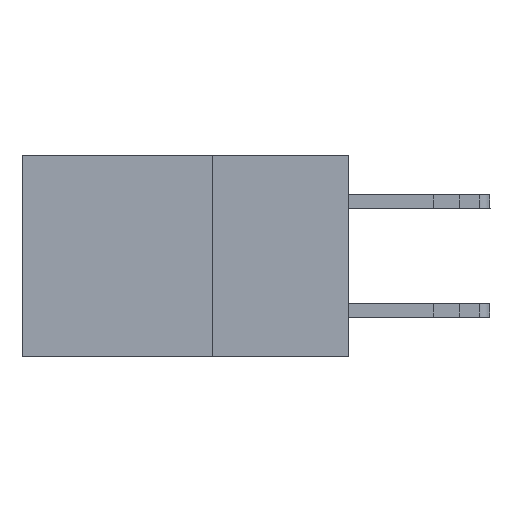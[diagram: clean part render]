
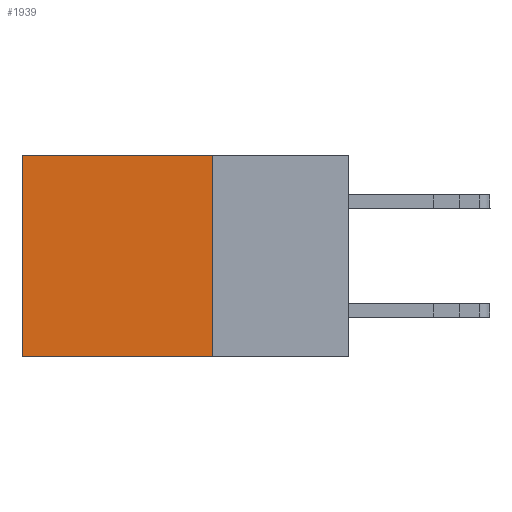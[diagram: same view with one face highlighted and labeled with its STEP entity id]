
A CAD part, left-side view. The second image highlights one B-rep face of the part: STEP entity #1939.
In plain terms, the highlighted planar face has unit normal (-1, 0, 0).
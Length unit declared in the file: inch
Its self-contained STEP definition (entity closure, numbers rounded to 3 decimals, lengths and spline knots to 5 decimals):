
#915 = CARTESIAN_POINT ( 'NONE',  ( 0.2615, 0.6, 0. ) ) ;
#1012 = VERTEX_POINT ( 'NONE', #915 ) ;
#1351 = DIRECTION ( 'NONE',  ( 0., 0., -1. ) ) ;
#1939 = ADVANCED_FACE ( 'NONE', ( #19668 ), #16979, .F. ) ;
#2074 = VECTOR ( 'NONE', #16151, 39.37008 ) ;
#2883 = CARTESIAN_POINT ( 'NONE',  ( 0.2615, 0.25, -0.37 ) ) ;
#3859 = ORIENTED_EDGE ( 'NONE', *, *, #13751, .T. ) ;
#4636 = ORIENTED_EDGE ( 'NONE', *, *, #5853, .F. ) ;
#4905 = AXIS2_PLACEMENT_3D ( 'NONE', #2883, #9135, #1351 ) ;
#5193 = CARTESIAN_POINT ( 'NONE',  ( 0.2615, 0.25, -0.37 ) ) ;
#5853 = EDGE_CURVE ( 'NONE', #20071, #15268, #13018, .T. ) ;
#5973 = CARTESIAN_POINT ( 'NONE',  ( 0.2615, 0.25, -0.37 ) ) ;
#6361 = CARTESIAN_POINT ( 'NONE',  ( 0.2615, 0.25, 0. ) ) ;
#9135 = DIRECTION ( 'NONE',  ( 1., 0., 0. ) ) ;
#9175 = EDGE_CURVE ( 'NONE', #15268, #10277, #20096, .T. ) ;
#10263 = CARTESIAN_POINT ( 'NONE',  ( 0.2615, 0.25, 0. ) ) ;
#10277 = VERTEX_POINT ( 'NONE', #17541 ) ;
#10577 = VECTOR ( 'NONE', #20102, 39.37008 ) ;
#10814 = CARTESIAN_POINT ( 'NONE',  ( 0.2615, 0.6, -0.37 ) ) ;
#11015 = ORIENTED_EDGE ( 'NONE', *, *, #16785, .T. ) ;
#11520 = LINE ( 'NONE', #6361, #2074 ) ;
#12437 = VECTOR ( 'NONE', #18556, 39.37008 ) ;
#13018 = LINE ( 'NONE', #5193, #17327 ) ;
#13751 = EDGE_CURVE ( 'NONE', #1012, #10277, #18565, .T. ) ;
#15268 = VERTEX_POINT ( 'NONE', #15750 ) ;
#15750 = CARTESIAN_POINT ( 'NONE',  ( 0.2615, 0.25, -0.37 ) ) ;
#16151 = DIRECTION ( 'NONE',  ( 0., 1., 0. ) ) ;
#16785 = EDGE_CURVE ( 'NONE', #20071, #1012, #11520, .T. ) ;
#16979 = PLANE ( 'NONE',  #4905 ) ;
#17327 = VECTOR ( 'NONE', #17760, 39.37008 ) ;
#17358 = EDGE_LOOP ( 'NONE', ( #3859, #17936, #4636, #11015 ) ) ;
#17541 = CARTESIAN_POINT ( 'NONE',  ( 0.2615, 0.6, -0.37 ) ) ;
#17760 = DIRECTION ( 'NONE',  ( 0., 0., -1. ) ) ;
#17936 = ORIENTED_EDGE ( 'NONE', *, *, #9175, .F. ) ;
#18556 = DIRECTION ( 'NONE',  ( 0., 1., 0. ) ) ;
#18565 = LINE ( 'NONE', #10814, #10577 ) ;
#19668 = FACE_OUTER_BOUND ( 'NONE', #17358, .T. ) ;
#20071 = VERTEX_POINT ( 'NONE', #10263 ) ;
#20096 = LINE ( 'NONE', #5973, #12437 ) ;
#20102 = DIRECTION ( 'NONE',  ( 0., 0., -1. ) ) ;
